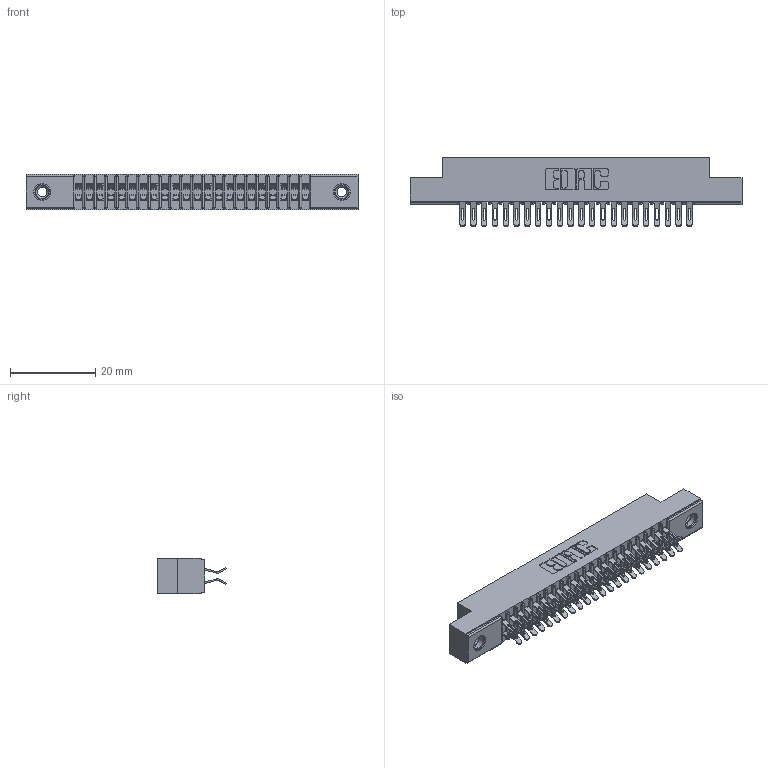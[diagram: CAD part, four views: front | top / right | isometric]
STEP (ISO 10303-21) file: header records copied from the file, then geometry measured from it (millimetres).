
FILE_DESCRIPTION (( 'STEP AP203' ), '1' );
FILE_NAME ('391-044-555-208.STEP', '2018-08-09T02:42:05', ( '' ), ( '' ), 'SwSTEP 2.0', 'SolidWorks 2016', '' );
FILE_SCHEMA (( 'CONFIG_CONTROL_DESIGN' ));
Length unit declared in the file: inch
Products named in the file (4): 341 Part_.156 (3.96) Dia Mounting Holes; 341-292-001_341-292-155; 345-250-001_345-250-003-102; 391-044-555-208
Assembly tree (47 placements, depth 2):
  391-044-555-208
    341 Part_.156 (3.96) Dia Mounting Holes
    341-292-001_341-292-155  x44
    345-250-001_345-250-003-102  x2
Bounding box: 78.11 x 16.31 x 8.38 mm (x, y, z)
Volume: 4496 mm3; surface area: 9726.7 mm2
Topology: 47 solids, 47 shells, 3608 faces, 10726 edges, 6978 vertices
Faces by surface type: plane 1948, cylinder 1556, sphere 46, torus 46, cone 12
Entity records: 30944 total; most frequent: CARTESIAN_POINT 5143, ORIENTED_EDGE 5092, DIRECTION 5006, EDGE_CURVE 2546, LINE 2016, VECTOR 2016, VERTEX_POINT 1616, AXIS2_PLACEMENT_3D 1495
